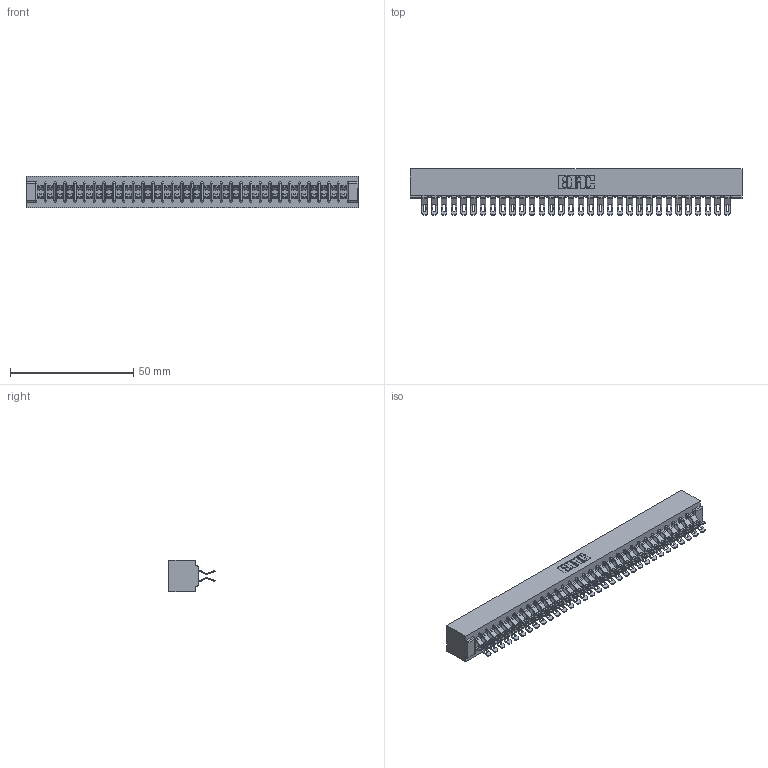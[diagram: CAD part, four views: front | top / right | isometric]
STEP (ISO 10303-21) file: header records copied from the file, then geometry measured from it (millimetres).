
FILE_DESCRIPTION (( 'STEP AP203' ), '1' );
FILE_NAME ('307-064-555-201.STEP', '2019-09-06T16:55:01', ( '' ), ( '' ), 'SwSTEP 2.0', 'SolidWorks 2016', '' );
FILE_SCHEMA (( 'CONFIG_CONTROL_DESIGN' ));
Length unit declared in the file: inch
Products named in the file (3): 307-064-555-201; 307-290-001_555; 307 Part_No Mounting Lugs
Assembly tree (65 placements, depth 2):
  307-064-555-201
    307 Part_No Mounting Lugs
    307-290-001_555  x64
Bounding box: 134.67 x 18.75 x 12.7 mm (x, y, z)
Volume: 14988 mm3; surface area: 19510.1 mm2
Topology: 65 solids, 65 shells, 4047 faces, 11883 edges, 7746 vertices
Faces by surface type: plane 2242, cylinder 1739, sphere 66
Entity records: 29949 total; most frequent: CARTESIAN_POINT 4904, ORIENTED_EDGE 4860, DIRECTION 4814, EDGE_CURVE 2430, VECTOR 1850, LINE 1850, VERTEX_POINT 1572, AXIS2_PLACEMENT_3D 1482
